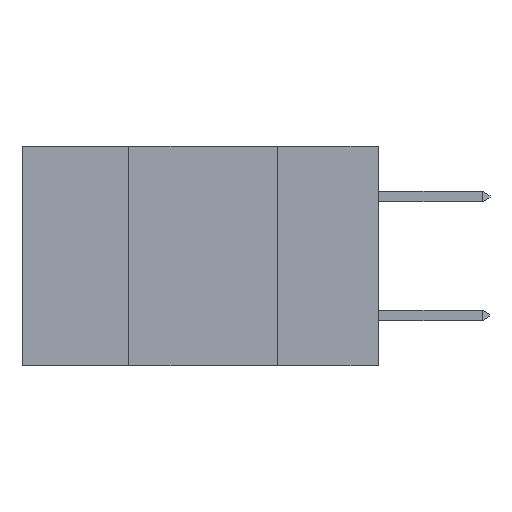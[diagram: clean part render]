
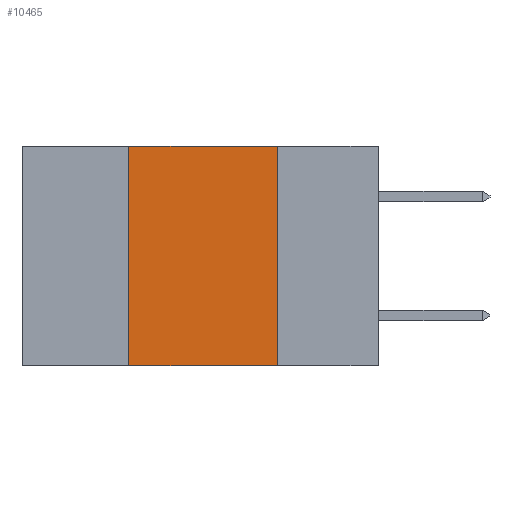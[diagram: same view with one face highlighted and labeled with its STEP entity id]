
A CAD part, left-side view. The second image highlights one B-rep face of the part: STEP entity #10465.
In plain terms, the highlighted planar face has unit normal (-1, 0, 0).
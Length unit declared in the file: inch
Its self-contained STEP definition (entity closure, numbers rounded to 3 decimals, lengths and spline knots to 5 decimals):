
#53 = LINE ( 'NONE', #2973, #4709 ) ;
#135 = VECTOR ( 'NONE', #11061, 39.37008 ) ;
#766 = EDGE_CURVE ( 'NONE', #1597, #1571, #53, .T. ) ;
#1013 = CARTESIAN_POINT ( 'NONE',  ( 0., 0.6, 0. ) ) ;
#1571 = VERTEX_POINT ( 'NONE', #8867 ) ;
#1597 = VERTEX_POINT ( 'NONE', #6163 ) ;
#1974 = DIRECTION ( 'NONE',  ( 1., 0., 0. ) ) ;
#2892 = DIRECTION ( 'NONE',  ( 0., 0., 1. ) ) ;
#2939 = CARTESIAN_POINT ( 'NONE',  ( 0., 0.17, -0.37 ) ) ;
#2973 = CARTESIAN_POINT ( 'NONE',  ( 0., 0.6, 0. ) ) ;
#3062 = DIRECTION ( 'NONE',  ( 0., -1., 0. ) ) ;
#3128 = VECTOR ( 'NONE', #7177, 39.37008 ) ;
#3259 = CARTESIAN_POINT ( 'NONE',  ( 0., 0.17, 0. ) ) ;
#3268 = LINE ( 'NONE', #8178, #7970 ) ;
#3705 = FACE_OUTER_BOUND ( 'NONE', #8438, .T. ) ;
#4005 = LINE ( 'NONE', #10610, #3128 ) ;
#4174 = EDGE_CURVE ( 'NONE', #11178, #8780, #4005, .T. ) ;
#4200 = ORIENTED_EDGE ( 'NONE', *, *, #8355, .F. ) ;
#4390 = ORIENTED_EDGE ( 'NONE', *, *, #766, .F. ) ;
#4709 = VECTOR ( 'NONE', #3062, 39.37008 ) ;
#4892 = AXIS2_PLACEMENT_3D ( 'NONE', #1013, #1974, #8191 ) ;
#5078 = LINE ( 'NONE', #3259, #135 ) ;
#5760 = CARTESIAN_POINT ( 'NONE',  ( 0., 0.42, -0.37 ) ) ;
#6163 = CARTESIAN_POINT ( 'NONE',  ( 0., 0.42, 0. ) ) ;
#6528 = PLANE ( 'NONE',  #4892 ) ;
#6759 = ORIENTED_EDGE ( 'NONE', *, *, #9371, .F. ) ;
#7177 = DIRECTION ( 'NONE',  ( 0., -1., 0. ) ) ;
#7970 = VECTOR ( 'NONE', #2892, 39.37008 ) ;
#7974 = ORIENTED_EDGE ( 'NONE', *, *, #4174, .T. ) ;
#8178 = CARTESIAN_POINT ( 'NONE',  ( 0., 0.42, 0. ) ) ;
#8191 = DIRECTION ( 'NONE',  ( 0., 0., -1. ) ) ;
#8355 = EDGE_CURVE ( 'NONE', #1571, #8780, #5078, .T. ) ;
#8438 = EDGE_LOOP ( 'NONE', ( #4200, #4390, #6759, #7974 ) ) ;
#8780 = VERTEX_POINT ( 'NONE', #2939 ) ;
#8867 = CARTESIAN_POINT ( 'NONE',  ( 0., 0.17, 0. ) ) ;
#9371 = EDGE_CURVE ( 'NONE', #11178, #1597, #3268, .T. ) ;
#10465 = ADVANCED_FACE ( 'NONE', ( #3705 ), #6528, .F. ) ;
#10610 = CARTESIAN_POINT ( 'NONE',  ( 0., 0.6, -0.37 ) ) ;
#11061 = DIRECTION ( 'NONE',  ( 0., 0., -1. ) ) ;
#11178 = VERTEX_POINT ( 'NONE', #5760 ) ;
